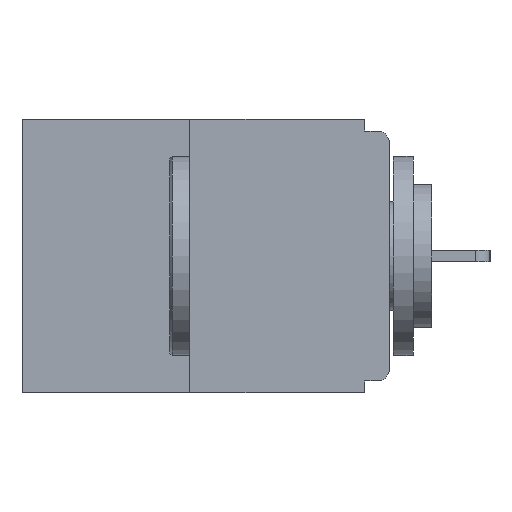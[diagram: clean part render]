
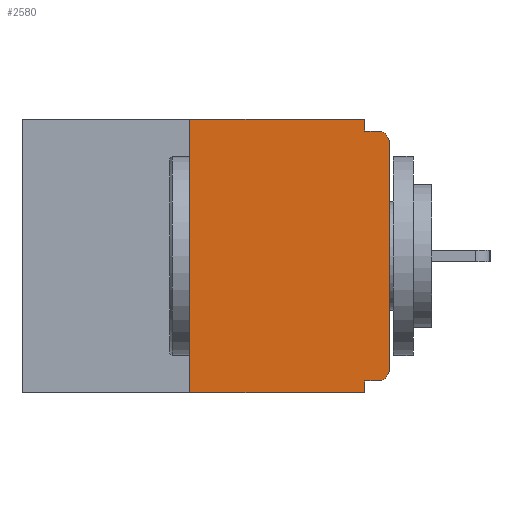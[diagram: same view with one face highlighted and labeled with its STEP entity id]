
A CAD part, left-side view. The second image highlights one B-rep face of the part: STEP entity #2580.
In plain terms, the highlighted planar face has unit normal (-1, 0, 0).
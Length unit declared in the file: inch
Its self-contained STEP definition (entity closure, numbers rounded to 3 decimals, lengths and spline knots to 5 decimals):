
#374 = LINE ( 'NONE', #12198, #8445 ) ;
#867 = EDGE_CURVE ( 'NONE', #6832, #6853, #12234, .T. ) ;
#879 = ORIENTED_EDGE ( 'NONE', *, *, #6615, .F. ) ;
#898 = VERTEX_POINT ( 'NONE', #1594 ) ;
#1568 = VERTEX_POINT ( 'NONE', #12953 ) ;
#1594 = CARTESIAN_POINT ( 'NONE',  ( 0., 0.25, -0.343 ) ) ;
#1617 = VERTEX_POINT ( 'NONE', #12872 ) ;
#1830 = DIRECTION ( 'NONE',  ( 0., 0., -1. ) ) ;
#1973 = CARTESIAN_POINT ( 'NONE',  ( 0., 0.031, -0.343 ) ) ;
#2042 = ORIENTED_EDGE ( 'NONE', *, *, #6796, .F. ) ;
#2385 = LINE ( 'NONE', #8624, #10439 ) ;
#2580 = ADVANCED_FACE ( 'NONE', ( #11758 ), #5816, .F. ) ;
#2635 = EDGE_CURVE ( 'NONE', #7965, #11822, #374, .T. ) ;
#2867 = VERTEX_POINT ( 'NONE', #6454 ) ;
#2934 = VECTOR ( 'NONE', #13422, 39.37008 ) ;
#3032 = CIRCLE ( 'NONE', #12522, 0.015 ) ;
#3041 = CARTESIAN_POINT ( 'NONE',  ( 0., 0.031, -0.343 ) ) ;
#3625 = AXIS2_PLACEMENT_3D ( 'NONE', #11003, #11067, #8536 ) ;
#3782 = DIRECTION ( 'NONE',  ( 0., 0., -1. ) ) ;
#3927 = ORIENTED_EDGE ( 'NONE', *, *, #11736, .F. ) ;
#3939 = DIRECTION ( 'NONE',  ( -1., 0., 0. ) ) ;
#3974 = CARTESIAN_POINT ( 'NONE',  ( 0., 0.015, -0.03 ) ) ;
#4105 = AXIS2_PLACEMENT_3D ( 'NONE', #5155, #13284, #11998 ) ;
#4276 = ORIENTED_EDGE ( 'NONE', *, *, #867, .T. ) ;
#4487 = CARTESIAN_POINT ( 'NONE',  ( 0., 0.031, -0.015 ) ) ;
#4612 = ORIENTED_EDGE ( 'NONE', *, *, #8459, .T. ) ;
#5155 = CARTESIAN_POINT ( 'NONE',  ( 0., 0.46, 0. ) ) ;
#5217 = DIRECTION ( 'NONE',  ( 0., 0., 1. ) ) ;
#5453 = CARTESIAN_POINT ( 'NONE',  ( 0., 0.25, 0. ) ) ;
#5816 = PLANE ( 'NONE',  #4105 ) ;
#6020 = EDGE_CURVE ( 'NONE', #6832, #6753, #10923, .T. ) ;
#6244 = CARTESIAN_POINT ( 'NONE',  ( 0., 0., -0.313 ) ) ;
#6299 = CARTESIAN_POINT ( 'NONE',  ( 0., 0.015, -0.328 ) ) ;
#6454 = CARTESIAN_POINT ( 'NONE',  ( 0., 0., -0.03 ) ) ;
#6615 = EDGE_CURVE ( 'NONE', #1617, #7965, #2385, .T. ) ;
#6622 = DIRECTION ( 'NONE',  ( 0., -1., 0. ) ) ;
#6624 = CARTESIAN_POINT ( 'NONE',  ( 0., 0., -0.015 ) ) ;
#6651 = VECTOR ( 'NONE', #11123, 39.37008 ) ;
#6753 = VERTEX_POINT ( 'NONE', #7270 ) ;
#6764 = ORIENTED_EDGE ( 'NONE', *, *, #11049, .T. ) ;
#6796 = EDGE_CURVE ( 'NONE', #11822, #1568, #7590, .T. ) ;
#6832 = VERTEX_POINT ( 'NONE', #6299 ) ;
#6853 = VERTEX_POINT ( 'NONE', #6244 ) ;
#6967 = VECTOR ( 'NONE', #5217, 39.37008 ) ;
#7270 = CARTESIAN_POINT ( 'NONE',  ( 0., 0.031, -0.328 ) ) ;
#7590 = LINE ( 'NONE', #6624, #7912 ) ;
#7773 = ORIENTED_EDGE ( 'NONE', *, *, #2635, .F. ) ;
#7912 = VECTOR ( 'NONE', #6622, 39.37008 ) ;
#7965 = VERTEX_POINT ( 'NONE', #12135 ) ;
#8445 = VECTOR ( 'NONE', #12288, 39.37008 ) ;
#8459 = EDGE_CURVE ( 'NONE', #2867, #1568, #3032, .T. ) ;
#8498 = DIRECTION ( 'NONE',  ( 0., -1., 0. ) ) ;
#8536 = DIRECTION ( 'NONE',  ( 0., 0., -1. ) ) ;
#8624 = CARTESIAN_POINT ( 'NONE',  ( 0., 0.46, 0. ) ) ;
#8948 = LINE ( 'NONE', #13205, #11911 ) ;
#9124 = LINE ( 'NONE', #1973, #11472 ) ;
#9403 = LINE ( 'NONE', #11233, #6651 ) ;
#9513 = ORIENTED_EDGE ( 'NONE', *, *, #10387, .F. ) ;
#9713 = LINE ( 'NONE', #5453, #6967 ) ;
#10387 = EDGE_CURVE ( 'NONE', #6753, #11935, #9124, .T. ) ;
#10439 = VECTOR ( 'NONE', #8498, 39.37008 ) ;
#10923 = LINE ( 'NONE', #13389, #2934 ) ;
#11003 = CARTESIAN_POINT ( 'NONE',  ( 0., 0.015, -0.313 ) ) ;
#11049 = EDGE_CURVE ( 'NONE', #898, #11935, #8948, .T. ) ;
#11067 = DIRECTION ( 'NONE',  ( -1., 0., 0. ) ) ;
#11123 = DIRECTION ( 'NONE',  ( 0., 0., 1. ) ) ;
#11233 = CARTESIAN_POINT ( 'NONE',  ( 0., 0., 0. ) ) ;
#11255 = EDGE_CURVE ( 'NONE', #6853, #2867, #9403, .T. ) ;
#11472 = VECTOR ( 'NONE', #1830, 39.37008 ) ;
#11736 = EDGE_CURVE ( 'NONE', #898, #1617, #9713, .T. ) ;
#11758 = FACE_OUTER_BOUND ( 'NONE', #13404, .T. ) ;
#11822 = VERTEX_POINT ( 'NONE', #4487 ) ;
#11911 = VECTOR ( 'NONE', #13154, 39.37008 ) ;
#11935 = VERTEX_POINT ( 'NONE', #3041 ) ;
#11998 = DIRECTION ( 'NONE',  ( 0., 0., -1. ) ) ;
#12135 = CARTESIAN_POINT ( 'NONE',  ( 0., 0.031, 0. ) ) ;
#12161 = ORIENTED_EDGE ( 'NONE', *, *, #6020, .F. ) ;
#12198 = CARTESIAN_POINT ( 'NONE',  ( 0., 0.031, 0. ) ) ;
#12234 = CIRCLE ( 'NONE', #3625, 0.015 ) ;
#12288 = DIRECTION ( 'NONE',  ( 0., 0., -1. ) ) ;
#12464 = ORIENTED_EDGE ( 'NONE', *, *, #11255, .T. ) ;
#12522 = AXIS2_PLACEMENT_3D ( 'NONE', #3974, #3939, #3782 ) ;
#12872 = CARTESIAN_POINT ( 'NONE',  ( 0., 0.25, 0. ) ) ;
#12953 = CARTESIAN_POINT ( 'NONE',  ( 0., 0.015, -0.015 ) ) ;
#13154 = DIRECTION ( 'NONE',  ( 0., -1., 0. ) ) ;
#13205 = CARTESIAN_POINT ( 'NONE',  ( 0., 0.46, -0.343 ) ) ;
#13284 = DIRECTION ( 'NONE',  ( 1., 0., 0. ) ) ;
#13389 = CARTESIAN_POINT ( 'NONE',  ( 0., 0., -0.328 ) ) ;
#13404 = EDGE_LOOP ( 'NONE', ( #879, #3927, #6764, #9513, #12161, #4276, #12464, #4612, #2042, #7773 ) ) ;
#13422 = DIRECTION ( 'NONE',  ( 0., 1., 0. ) ) ;
